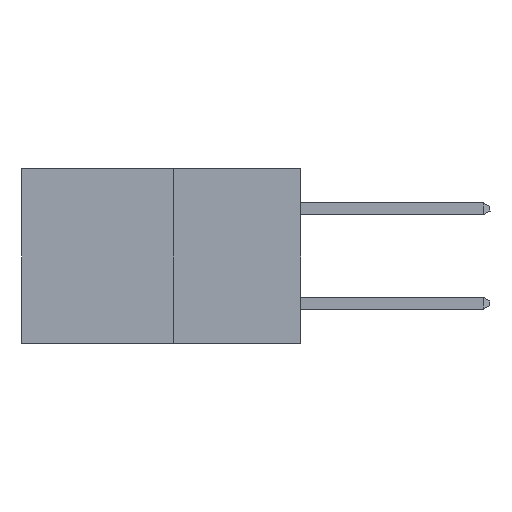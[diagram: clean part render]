
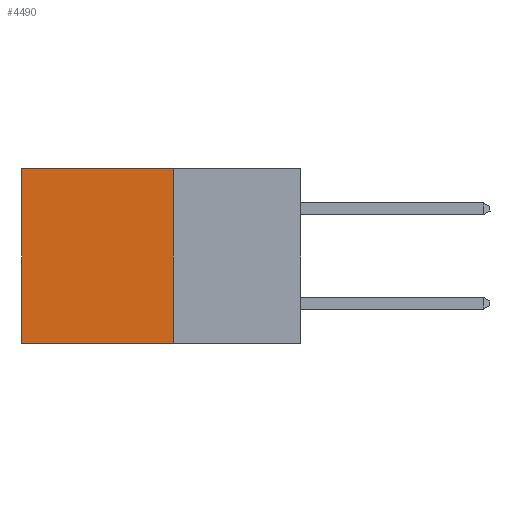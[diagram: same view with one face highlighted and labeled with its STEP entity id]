
A CAD part, left-side view. The second image highlights one B-rep face of the part: STEP entity #4490.
In plain terms, the highlighted planar face has unit normal (-1, 0, 0).
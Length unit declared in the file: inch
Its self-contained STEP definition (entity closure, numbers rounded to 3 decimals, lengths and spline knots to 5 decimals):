
#202 = CARTESIAN_POINT ( 'NONE',  ( 0.277, 0.59, 0. ) ) ;
#734 = VECTOR ( 'NONE', #17252, 39.37008 ) ;
#1011 = EDGE_CURVE ( 'NONE', #21209, #11363, #3437, .T. ) ;
#1980 = ORIENTED_EDGE ( 'NONE', *, *, #11073, .F. ) ;
#2124 = DIRECTION ( 'NONE',  ( 0., 1., 0. ) ) ;
#2513 = CARTESIAN_POINT ( 'NONE',  ( 0.277, 0.27, 0. ) ) ;
#3351 = ORIENTED_EDGE ( 'NONE', *, *, #13197, .T. ) ;
#3437 = LINE ( 'NONE', #3580, #13994 ) ;
#3580 = CARTESIAN_POINT ( 'NONE',  ( 0.277, 0.27, -0.37 ) ) ;
#4354 = ORIENTED_EDGE ( 'NONE', *, *, #23117, .T. ) ;
#4490 = ADVANCED_FACE ( 'NONE', ( #22287 ), #21129, .F. ) ;
#5207 = LINE ( 'NONE', #11475, #734 ) ;
#5611 = CARTESIAN_POINT ( 'NONE',  ( 0.277, 0.27, -0.37 ) ) ;
#9046 = EDGE_LOOP ( 'NONE', ( #4354, #14455, #1980, #3351 ) ) ;
#10539 = VERTEX_POINT ( 'NONE', #14314 ) ;
#10556 = LINE ( 'NONE', #19435, #14510 ) ;
#11073 = EDGE_CURVE ( 'NONE', #10539, #21209, #10556, .T. ) ;
#11363 = VERTEX_POINT ( 'NONE', #22024 ) ;
#11475 = CARTESIAN_POINT ( 'NONE',  ( 0.277, 0.59, -0.37 ) ) ;
#13031 = AXIS2_PLACEMENT_3D ( 'NONE', #16191, #24338, #24152 ) ;
#13197 = EDGE_CURVE ( 'NONE', #10539, #21375, #22610, .T. ) ;
#13994 = VECTOR ( 'NONE', #2124, 39.37008 ) ;
#14314 = CARTESIAN_POINT ( 'NONE',  ( 0.277, 0.27, 0. ) ) ;
#14441 = VECTOR ( 'NONE', #16294, 39.37008 ) ;
#14455 = ORIENTED_EDGE ( 'NONE', *, *, #1011, .F. ) ;
#14510 = VECTOR ( 'NONE', #21323, 39.37008 ) ;
#16191 = CARTESIAN_POINT ( 'NONE',  ( 0.277, 0.27, -0.37 ) ) ;
#16294 = DIRECTION ( 'NONE',  ( 0., 1., 0. ) ) ;
#17252 = DIRECTION ( 'NONE',  ( 0., 0., -1. ) ) ;
#19435 = CARTESIAN_POINT ( 'NONE',  ( 0.277, 0.27, -0.37 ) ) ;
#21129 = PLANE ( 'NONE',  #13031 ) ;
#21209 = VERTEX_POINT ( 'NONE', #5611 ) ;
#21323 = DIRECTION ( 'NONE',  ( 0., 0., -1. ) ) ;
#21375 = VERTEX_POINT ( 'NONE', #202 ) ;
#22024 = CARTESIAN_POINT ( 'NONE',  ( 0.277, 0.59, -0.37 ) ) ;
#22287 = FACE_OUTER_BOUND ( 'NONE', #9046, .T. ) ;
#22610 = LINE ( 'NONE', #2513, #14441 ) ;
#23117 = EDGE_CURVE ( 'NONE', #21375, #11363, #5207, .T. ) ;
#24152 = DIRECTION ( 'NONE',  ( 0., 0., -1. ) ) ;
#24338 = DIRECTION ( 'NONE',  ( 1., 0., 0. ) ) ;
